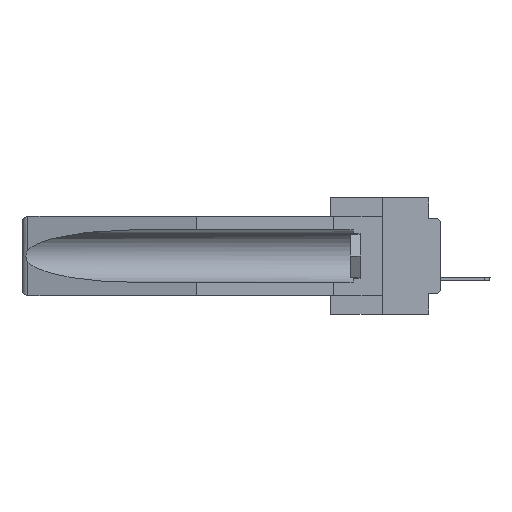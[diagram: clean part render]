
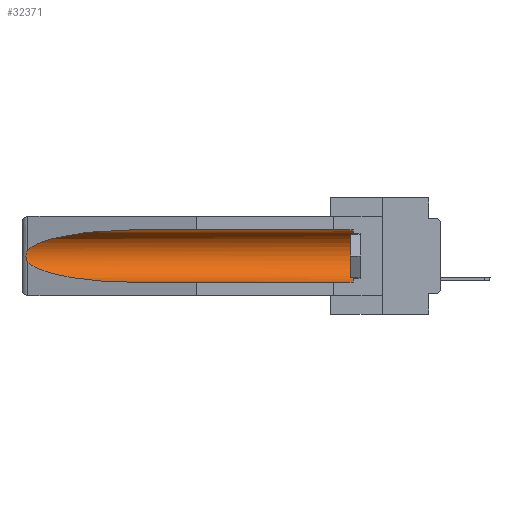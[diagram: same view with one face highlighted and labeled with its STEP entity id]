
A CAD part, left-side view. The second image highlights one B-rep face of the part: STEP entity #32371.
In plain terms, the highlighted cylindrical face has radius 2.857 mm (diameter 5.715 mm), a partial arc.
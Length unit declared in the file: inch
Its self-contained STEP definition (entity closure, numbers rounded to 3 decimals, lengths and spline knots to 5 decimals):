
#9 = VERTEX_POINT ( 'NONE', #30311 ) ;
#38 = DIRECTION ( 'NONE',  ( 0., 1., 0. ) ) ;
#537 = DIRECTION ( 'NONE',  ( 0., 0., 1. ) ) ;
#1221 = EDGE_CURVE ( 'NONE', #23070, #17884, #29770, .T. ) ;
#2280 = CARTESIAN_POINT ( 'NONE',  ( 0.25451, 1.48313, -0.24835 ) ) ;
#2835 = CARTESIAN_POINT ( 'NONE',  ( 0.26654, 1.53092, -0.15636 ) ) ;
#3869 = CARTESIAN_POINT ( 'NONE',  ( 0.155, 0.126, -0.059 ) ) ;
#4080 = CARTESIAN_POINT ( 'NONE',  ( 0.155, 1.07973, -0.059 ) ) ;
#5445 = CARTESIAN_POINT ( 'NONE',  ( 0.155, 1.07973, -0.284 ) ) ;
#6681 = CARTESIAN_POINT ( 'NONE',  ( 0.26537, 1.52718, -0.19328 ) ) ;
#7064 = EDGE_CURVE ( 'NONE', #22983, #9, #11977, .T. ) ;
#7579 = CARTESIAN_POINT ( 'NONE',  ( 0.26537, 1.52718, -0.19328 ) ) ;
#8130 = AXIS2_PLACEMENT_3D ( 'NONE', #26541, #31815, #31695 ) ;
#8229 = CARTESIAN_POINT ( 'NONE',  ( 0.26537, 1.52718, -0.19328 ) ) ;
#8466 = CARTESIAN_POINT ( 'NONE',  ( 0.2675, 1.53308, -0.16763 ) ) ;
#8842 = CYLINDRICAL_SURFACE ( 'NONE', #8130, 0.1125 ) ;
#9131 = ORIENTED_EDGE ( 'NONE', *, *, #7064, .T. ) ;
#10054 = LINE ( 'NONE', #16107, #18414 ) ;
#10815 = ORIENTED_EDGE ( 'NONE', *, *, #30795, .T. ) ;
#11977 =( BOUNDED_CURVE ( )  B_SPLINE_CURVE ( 3, ( #7579, #2280, #21476, #5445 ),
 .UNSPECIFIED., .F., .T. ) 
 B_SPLINE_CURVE_WITH_KNOTS ( ( 4, 4 ),
 ( 0.1948, 1.5708 ),
 .UNSPECIFIED. ) 
 CURVE ( )  GEOMETRIC_REPRESENTATION_ITEM ( )  RATIONAL_B_SPLINE_CURVE ( ( 1., 0.848, 0.848, 1. ) ) 
 REPRESENTATION_ITEM ( '' )  );
#12501 = LINE ( 'NONE', #31027, #26307 ) ;
#12634 = B_SPLINE_CURVE_WITH_KNOTS ( 'NONE', 3,
 ( #32273, #24387, #2835, #27095, #8466, #24493, #24284, #32492, #16418, #8229 ),
 .UNSPECIFIED., .F., .F.,
 ( 4, 2, 2, 2, 4 ),
 ( 0., 0.00029, 0.00058, 0.00087, 0.00117 ),
 .UNSPECIFIED. ) ;
#13019 = CARTESIAN_POINT ( 'NONE',  ( 0.155, 1.07973, -0.059 ) ) ;
#13802 = CARTESIAN_POINT ( 'NONE',  ( 0.26537, 1.52718, -0.14972 ) ) ;
#14398 = CARTESIAN_POINT ( 'NONE',  ( 0.155, 0.126, -0.1715 ) ) ;
#15995 = FACE_OUTER_BOUND ( 'NONE', #23961, .T. ) ;
#16107 = CARTESIAN_POINT ( 'NONE',  ( 0.155, -0.30754, -0.059 ) ) ;
#16418 = CARTESIAN_POINT ( 'NONE',  ( 0.26597, 1.5296, -0.19026 ) ) ;
#16636 = CIRCLE ( 'NONE', #26958, 0.1125 ) ;
#17884 = VERTEX_POINT ( 'NONE', #24522 ) ;
#18414 = VECTOR ( 'NONE', #38, 39.37008 ) ;
#18893 = ORIENTED_EDGE ( 'NONE', *, *, #1221, .T. ) ;
#19311 = DIRECTION ( 'NONE',  ( 0., -1., 0. ) ) ;
#19885 = ORIENTED_EDGE ( 'NONE', *, *, #25201, .F. ) ;
#21476 = CARTESIAN_POINT ( 'NONE',  ( 0.21114, 1.30732, -0.284 ) ) ;
#22790 = DIRECTION ( 'NONE',  ( 0., 1., 0. ) ) ;
#22983 = VERTEX_POINT ( 'NONE', #6681 ) ;
#23070 = VERTEX_POINT ( 'NONE', #4080 ) ;
#23961 = EDGE_LOOP ( 'NONE', ( #18893, #10815, #9131, #19885, #25609, #27188 ) ) ;
#24284 = CARTESIAN_POINT ( 'NONE',  ( 0.2673, 1.53269, -0.17917 ) ) ;
#24387 = CARTESIAN_POINT ( 'NONE',  ( 0.26597, 1.52961, -0.15275 ) ) ;
#24493 = CARTESIAN_POINT ( 'NONE',  ( 0.2675, 1.53308, -0.17534 ) ) ;
#24522 = CARTESIAN_POINT ( 'NONE',  ( 0.26537, 1.52718, -0.14972 ) ) ;
#25088 = EDGE_CURVE ( 'NONE', #26299, #30915, #16636, .T. ) ;
#25201 = EDGE_CURVE ( 'NONE', #26299, #9, #12501, .T. ) ;
#25609 = ORIENTED_EDGE ( 'NONE', *, *, #25088, .T. ) ;
#26299 = VERTEX_POINT ( 'NONE', #29779 ) ;
#26307 = VECTOR ( 'NONE', #22790, 39.37008 ) ;
#26541 = CARTESIAN_POINT ( 'NONE',  ( 0.155, -0.30754, -0.1715 ) ) ;
#26916 = CARTESIAN_POINT ( 'NONE',  ( 0.21114, 1.30732, -0.059 ) ) ;
#26958 = AXIS2_PLACEMENT_3D ( 'NONE', #14398, #19311, #537 ) ;
#27095 = CARTESIAN_POINT ( 'NONE',  ( 0.2673, 1.5327, -0.16383 ) ) ;
#27188 = ORIENTED_EDGE ( 'NONE', *, *, #27363, .T. ) ;
#27363 = EDGE_CURVE ( 'NONE', #30915, #23070, #10054, .T. ) ;
#29770 =( BOUNDED_CURVE ( )  B_SPLINE_CURVE ( 3, ( #13019, #26916, #29818, #13802 ),
 .UNSPECIFIED., .F., .F. ) 
 B_SPLINE_CURVE_WITH_KNOTS ( ( 4, 4 ),
 ( 4.71239, 6.08839 ),
 .UNSPECIFIED. ) 
 CURVE ( )  GEOMETRIC_REPRESENTATION_ITEM ( )  RATIONAL_B_SPLINE_CURVE ( ( 1., 0.848, 0.848, 1. ) ) 
 REPRESENTATION_ITEM ( '' )  );
#29779 = CARTESIAN_POINT ( 'NONE',  ( 0.155, 0.126, -0.284 ) ) ;
#29818 = CARTESIAN_POINT ( 'NONE',  ( 0.25451, 1.48313, -0.09465 ) ) ;
#30311 = CARTESIAN_POINT ( 'NONE',  ( 0.155, 1.07973, -0.284 ) ) ;
#30795 = EDGE_CURVE ( 'NONE', #17884, #22983, #12634, .T. ) ;
#30915 = VERTEX_POINT ( 'NONE', #3869 ) ;
#31027 = CARTESIAN_POINT ( 'NONE',  ( 0.155, -0.30754, -0.284 ) ) ;
#31695 = DIRECTION ( 'NONE',  ( 0., 0., 1. ) ) ;
#31815 = DIRECTION ( 'NONE',  ( 0., 1., 0. ) ) ;
#32273 = CARTESIAN_POINT ( 'NONE',  ( 0.26537, 1.52718, -0.14972 ) ) ;
#32371 = ADVANCED_FACE ( 'NONE', ( #15995 ), #8842, .F. ) ;
#32492 = CARTESIAN_POINT ( 'NONE',  ( 0.26655, 1.53094, -0.18657 ) ) ;
